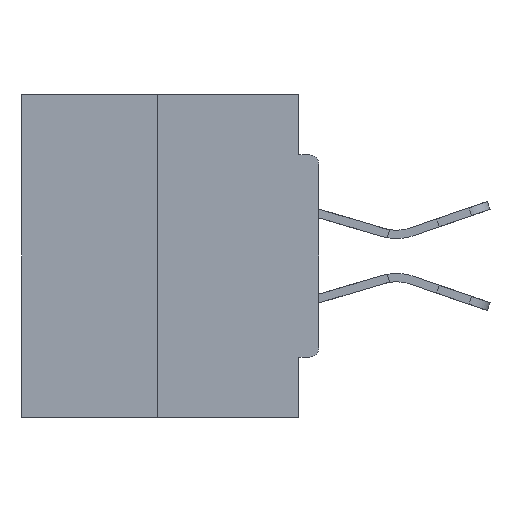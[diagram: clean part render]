
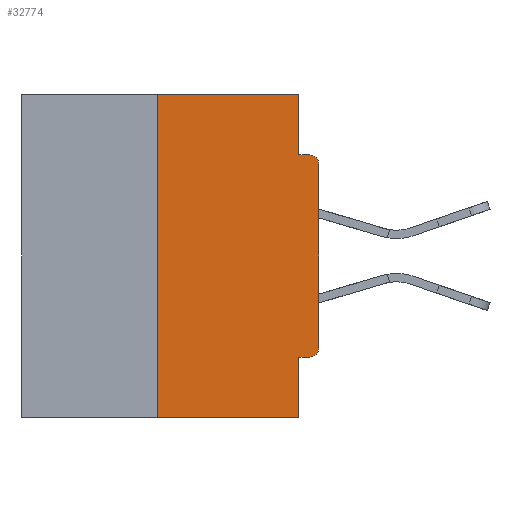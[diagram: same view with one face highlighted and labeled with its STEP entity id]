
A CAD part, left-side view. The second image highlights one B-rep face of the part: STEP entity #32774.
In plain terms, the highlighted planar face has unit normal (-1, 0, 0).
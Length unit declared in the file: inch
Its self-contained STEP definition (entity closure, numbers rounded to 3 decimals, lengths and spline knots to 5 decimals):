
#305 = CARTESIAN_POINT ( 'NONE',  ( 0., 0., -0.1085 ) ) ;
#758 = VECTOR ( 'NONE', #47816, 39.37008 ) ;
#883 = LINE ( 'NONE', #17302, #34642 ) ;
#1381 = ORIENTED_EDGE ( 'NONE', *, *, #38576, .F. ) ;
#1807 = VERTEX_POINT ( 'NONE', #46794 ) ;
#1960 = CARTESIAN_POINT ( 'NONE',  ( 0., 0.031, -0.5 ) ) ;
#2457 = VERTEX_POINT ( 'NONE', #26260 ) ;
#4428 = FACE_OUTER_BOUND ( 'NONE', #27746, .T. ) ;
#5681 = CARTESIAN_POINT ( 'NONE',  ( 0., 0.015, -0.3915 ) ) ;
#5744 = DIRECTION ( 'NONE',  ( 0., -1., 0. ) ) ;
#6156 = ORIENTED_EDGE ( 'NONE', *, *, #21945, .T. ) ;
#6236 = DIRECTION ( 'NONE',  ( 0., 0., -1. ) ) ;
#6568 = DIRECTION ( 'NONE',  ( 1., 0., 0. ) ) ;
#6683 = DIRECTION ( 'NONE',  ( 0., 0., -1. ) ) ;
#6968 = EDGE_CURVE ( 'NONE', #11144, #12899, #26399, .T. ) ;
#7162 = AXIS2_PLACEMENT_3D ( 'NONE', #37129, #48265, #40705 ) ;
#9955 = CARTESIAN_POINT ( 'NONE',  ( 0., 0.015, -0.0935 ) ) ;
#10369 = ORIENTED_EDGE ( 'NONE', *, *, #40399, .F. ) ;
#10559 = LINE ( 'NONE', #42833, #15207 ) ;
#11129 = ORIENTED_EDGE ( 'NONE', *, *, #6968, .F. ) ;
#11144 = VERTEX_POINT ( 'NONE', #15815 ) ;
#11446 = CARTESIAN_POINT ( 'NONE',  ( 0., 0., -0.0935 ) ) ;
#12536 = EDGE_CURVE ( 'NONE', #37571, #1807, #17711, .T. ) ;
#12899 = VERTEX_POINT ( 'NONE', #37430 ) ;
#13639 = VERTEX_POINT ( 'NONE', #1960 ) ;
#14924 = CIRCLE ( 'NONE', #25711, 0.015 ) ;
#15207 = VECTOR ( 'NONE', #6683, 39.37008 ) ;
#15815 = CARTESIAN_POINT ( 'NONE',  ( 0., 0.015, -0.4065 ) ) ;
#17036 = VERTEX_POINT ( 'NONE', #22139 ) ;
#17302 = CARTESIAN_POINT ( 'NONE',  ( 0., 0.46, -0.5 ) ) ;
#17318 = CARTESIAN_POINT ( 'NONE',  ( 0., 0.46, 0. ) ) ;
#17711 = LINE ( 'NONE', #36446, #42229 ) ;
#18028 = ORIENTED_EDGE ( 'NONE', *, *, #12536, .F. ) ;
#21642 = ORIENTED_EDGE ( 'NONE', *, *, #26163, .F. ) ;
#21945 = EDGE_CURVE ( 'NONE', #37571, #13639, #883, .T. ) ;
#22139 = CARTESIAN_POINT ( 'NONE',  ( 0., 0.031, -0.0935 ) ) ;
#22191 = AXIS2_PLACEMENT_3D ( 'NONE', #17318, #6568, #6236 ) ;
#22207 = ORIENTED_EDGE ( 'NONE', *, *, #47594, .F. ) ;
#22984 = CARTESIAN_POINT ( 'NONE',  ( 0., 0.031, 0. ) ) ;
#24749 = ORIENTED_EDGE ( 'NONE', *, *, #32809, .T. ) ;
#25711 = AXIS2_PLACEMENT_3D ( 'NONE', #5681, #31441, #42667 ) ;
#26163 = EDGE_CURVE ( 'NONE', #17036, #44189, #27239, .T. ) ;
#26260 = CARTESIAN_POINT ( 'NONE',  ( 0., 0., -0.3915 ) ) ;
#26399 = LINE ( 'NONE', #28913, #46217 ) ;
#27033 = EDGE_CURVE ( 'NONE', #11144, #2457, #14924, .T. ) ;
#27061 = VECTOR ( 'NONE', #41883, 39.37008 ) ;
#27239 = LINE ( 'NONE', #11446, #44141 ) ;
#27746 = EDGE_LOOP ( 'NONE', ( #22207, #18028, #6156, #1381, #11129, #39341, #24749, #33692, #21642, #10369 ) ) ;
#28913 = CARTESIAN_POINT ( 'NONE',  ( 0., 0., -0.4065 ) ) ;
#28929 = DIRECTION ( 'NONE',  ( 0., 0., 1. ) ) ;
#30574 = CIRCLE ( 'NONE', #7162, 0.015 ) ;
#31441 = DIRECTION ( 'NONE',  ( -1., 0., 0. ) ) ;
#32156 = PLANE ( 'NONE',  #22191 ) ;
#32774 = ADVANCED_FACE ( 'NONE', ( #4428 ), #32156, .F. ) ;
#32809 = EDGE_CURVE ( 'NONE', #2457, #47776, #34153, .T. ) ;
#33692 = ORIENTED_EDGE ( 'NONE', *, *, #39995, .T. ) ;
#34153 = LINE ( 'NONE', #43381, #41163 ) ;
#34642 = VECTOR ( 'NONE', #5744, 39.37008 ) ;
#36191 = CARTESIAN_POINT ( 'NONE',  ( 0., 0.25, -0.5 ) ) ;
#36425 = DIRECTION ( 'NONE',  ( 0., 1., 0. ) ) ;
#36442 = CARTESIAN_POINT ( 'NONE',  ( 0., 0.46, 0. ) ) ;
#36446 = CARTESIAN_POINT ( 'NONE',  ( 0., 0.25, 0. ) ) ;
#37129 = CARTESIAN_POINT ( 'NONE',  ( 0., 0.015, -0.1085 ) ) ;
#37430 = CARTESIAN_POINT ( 'NONE',  ( 0., 0.031, -0.4065 ) ) ;
#37571 = VERTEX_POINT ( 'NONE', #36191 ) ;
#38576 = EDGE_CURVE ( 'NONE', #12899, #13639, #10559, .T. ) ;
#38687 = LINE ( 'NONE', #22984, #27061 ) ;
#39284 = VERTEX_POINT ( 'NONE', #41937 ) ;
#39341 = ORIENTED_EDGE ( 'NONE', *, *, #27033, .T. ) ;
#39995 = EDGE_CURVE ( 'NONE', #47776, #44189, #30574, .T. ) ;
#40399 = EDGE_CURVE ( 'NONE', #39284, #17036, #38687, .T. ) ;
#40705 = DIRECTION ( 'NONE',  ( 0., 0., -1. ) ) ;
#41163 = VECTOR ( 'NONE', #43536, 39.37008 ) ;
#41883 = DIRECTION ( 'NONE',  ( 0., 0., -1. ) ) ;
#41937 = CARTESIAN_POINT ( 'NONE',  ( 0., 0.031, 0. ) ) ;
#42229 = VECTOR ( 'NONE', #28929, 39.37008 ) ;
#42667 = DIRECTION ( 'NONE',  ( 0., 0., -1. ) ) ;
#42833 = CARTESIAN_POINT ( 'NONE',  ( 0., 0.031, -0.5 ) ) ;
#43381 = CARTESIAN_POINT ( 'NONE',  ( 0., 0., 0. ) ) ;
#43536 = DIRECTION ( 'NONE',  ( 0., 0., 1. ) ) ;
#44141 = VECTOR ( 'NONE', #44808, 39.37008 ) ;
#44189 = VERTEX_POINT ( 'NONE', #9955 ) ;
#44808 = DIRECTION ( 'NONE',  ( 0., -1., 0. ) ) ;
#45571 = LINE ( 'NONE', #36442, #758 ) ;
#46217 = VECTOR ( 'NONE', #36425, 39.37008 ) ;
#46794 = CARTESIAN_POINT ( 'NONE',  ( 0., 0.25, 0. ) ) ;
#47594 = EDGE_CURVE ( 'NONE', #1807, #39284, #45571, .T. ) ;
#47776 = VERTEX_POINT ( 'NONE', #305 ) ;
#47816 = DIRECTION ( 'NONE',  ( 0., -1., 0. ) ) ;
#48265 = DIRECTION ( 'NONE',  ( -1., 0., 0. ) ) ;
